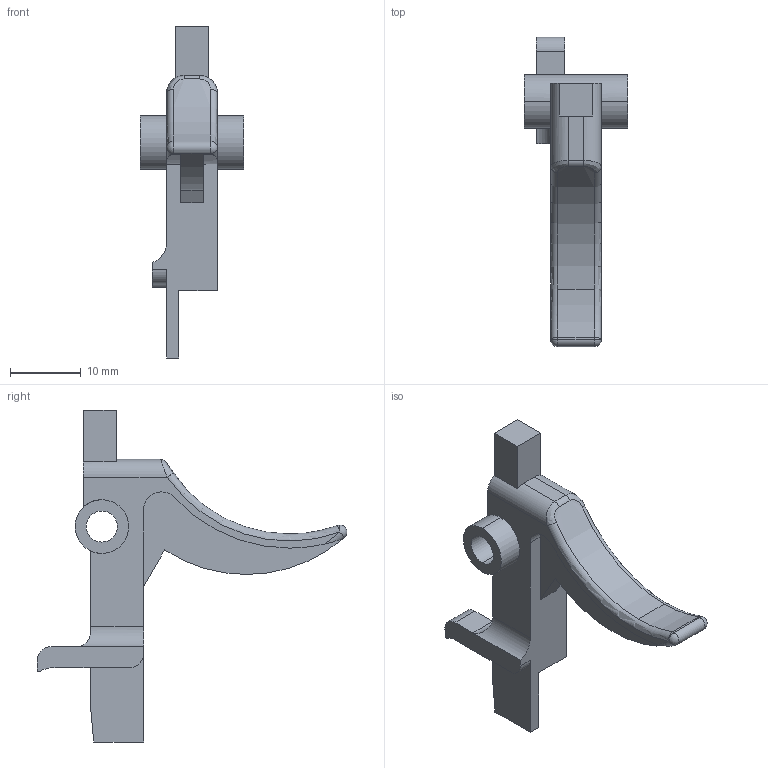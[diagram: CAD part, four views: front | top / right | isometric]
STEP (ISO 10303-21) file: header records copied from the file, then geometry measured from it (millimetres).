
FILE_DESCRIPTION (( 'STEP AP203' ), '1' );
FILE_NAME ('trigger.STEP', '2021-12-29T04:20:30', ( '' ), ( '' ), 'SwSTEP 2.0', 'SolidWorks 2015', '' );
FILE_SCHEMA (( 'CONFIG_CONTROL_DESIGN' ));
Length unit declared in the file: millimetre
Products named in the file (1): trigger
Bounding box: 14.6 x 43.87 x 47 mm (x, y, z)
Volume: 3239.9 mm3; surface area: 2614.1 mm2
Topology: 1 solids, 1 shells, 63 faces, 172 edges, 109 vertices
Faces by surface type: cylinder 27, plane 26, sphere 4, torus 4, bspline 2
Entity records: 2215 total; most frequent: CARTESIAN_POINT 522, DIRECTION 356, ORIENTED_EDGE 336, EDGE_CURVE 168, AXIS2_PLACEMENT_3D 133, VERTEX_POINT 107, VECTOR 90, LINE 90
